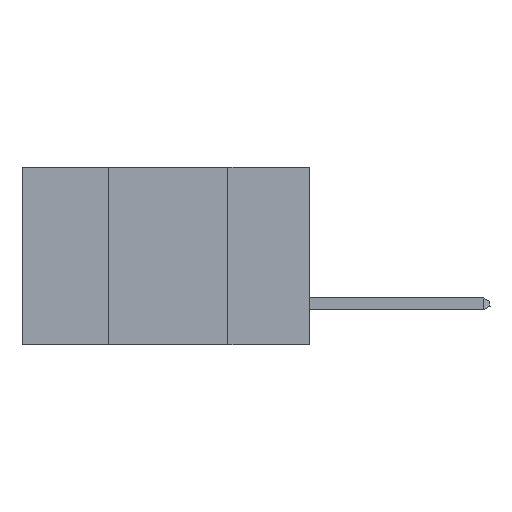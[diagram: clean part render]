
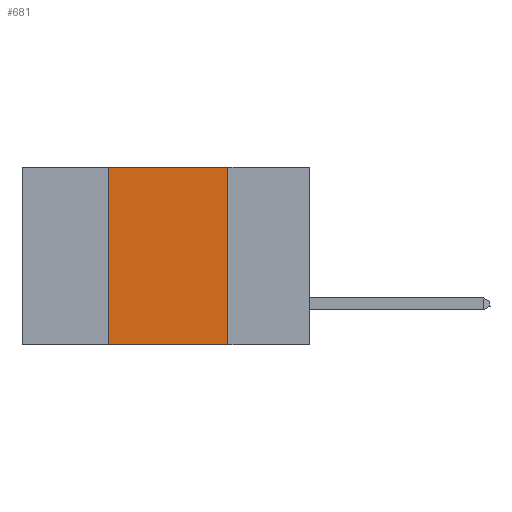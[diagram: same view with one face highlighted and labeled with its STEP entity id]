
A CAD part, left-side view. The second image highlights one B-rep face of the part: STEP entity #681.
In plain terms, the highlighted planar face has unit normal (-1, 0, 0).
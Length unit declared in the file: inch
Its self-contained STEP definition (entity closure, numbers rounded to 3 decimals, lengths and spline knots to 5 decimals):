
#140 = CARTESIAN_POINT ( 'NONE',  ( 0., 0.6, -0.37 ) ) ;
#201 = VECTOR ( 'NONE', #2535, 39.37008 ) ;
#681 = ADVANCED_FACE ( 'NONE', ( #3246 ), #10195, .F. ) ;
#750 = DIRECTION ( 'NONE',  ( 0., 0., 1. ) ) ;
#822 = EDGE_CURVE ( 'NONE', #3830, #3047, #9734, .T. ) ;
#935 = DIRECTION ( 'NONE',  ( 0., 0., -1. ) ) ;
#1369 = LINE ( 'NONE', #2006, #2874 ) ;
#2006 = CARTESIAN_POINT ( 'NONE',  ( 0., 0.42, 0. ) ) ;
#2089 = DIRECTION ( 'NONE',  ( 0., -1., 0. ) ) ;
#2139 = EDGE_CURVE ( 'NONE', #3842, #2260, #1369, .T. ) ;
#2260 = VERTEX_POINT ( 'NONE', #6445 ) ;
#2535 = DIRECTION ( 'NONE',  ( 0., -1., 0. ) ) ;
#2641 = VECTOR ( 'NONE', #2089, 39.37008 ) ;
#2874 = VECTOR ( 'NONE', #750, 39.37008 ) ;
#2963 = CARTESIAN_POINT ( 'NONE',  ( 0., 0.42, -0.37 ) ) ;
#3036 = LINE ( 'NONE', #140, #201 ) ;
#3047 = VERTEX_POINT ( 'NONE', #5170 ) ;
#3246 = FACE_OUTER_BOUND ( 'NONE', #5250, .T. ) ;
#3807 = CARTESIAN_POINT ( 'NONE',  ( 0., 0.6, 0. ) ) ;
#3830 = VERTEX_POINT ( 'NONE', #9488 ) ;
#3842 = VERTEX_POINT ( 'NONE', #2963 ) ;
#4218 = CARTESIAN_POINT ( 'NONE',  ( 0., 0.6, 0. ) ) ;
#4320 = ORIENTED_EDGE ( 'NONE', *, *, #9904, .T. ) ;
#4902 = DIRECTION ( 'NONE',  ( 1., 0., 0. ) ) ;
#5170 = CARTESIAN_POINT ( 'NONE',  ( 0., 0.17, -0.37 ) ) ;
#5250 = EDGE_LOOP ( 'NONE', ( #12703, #10363, #13755, #4320 ) ) ;
#5362 = VECTOR ( 'NONE', #935, 39.37008 ) ;
#5835 = DIRECTION ( 'NONE',  ( 0., 0., -1. ) ) ;
#6445 = CARTESIAN_POINT ( 'NONE',  ( 0., 0.42, 0. ) ) ;
#9385 = AXIS2_PLACEMENT_3D ( 'NONE', #3807, #4902, #5835 ) ;
#9488 = CARTESIAN_POINT ( 'NONE',  ( 0., 0.17, 0. ) ) ;
#9734 = LINE ( 'NONE', #12689, #5362 ) ;
#9904 = EDGE_CURVE ( 'NONE', #3842, #3047, #3036, .T. ) ;
#10195 = PLANE ( 'NONE',  #9385 ) ;
#10363 = ORIENTED_EDGE ( 'NONE', *, *, #10973, .F. ) ;
#10973 = EDGE_CURVE ( 'NONE', #2260, #3830, #13520, .T. ) ;
#12689 = CARTESIAN_POINT ( 'NONE',  ( 0., 0.17, 0. ) ) ;
#12703 = ORIENTED_EDGE ( 'NONE', *, *, #822, .F. ) ;
#13520 = LINE ( 'NONE', #4218, #2641 ) ;
#13755 = ORIENTED_EDGE ( 'NONE', *, *, #2139, .F. ) ;
